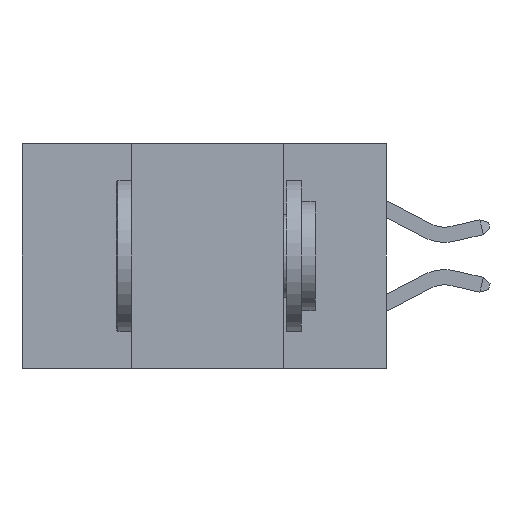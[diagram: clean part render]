
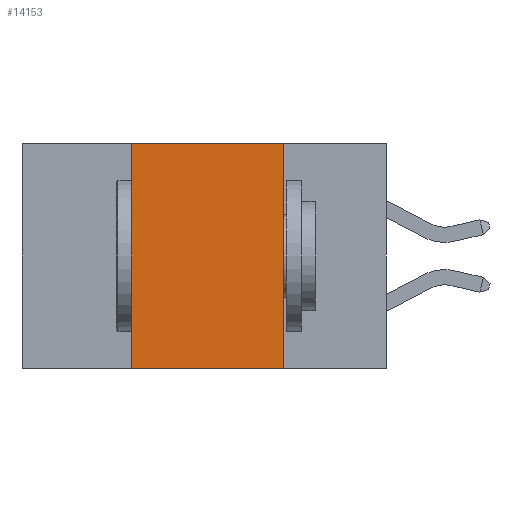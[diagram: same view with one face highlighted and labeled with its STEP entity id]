
A CAD part, left-side view. The second image highlights one B-rep face of the part: STEP entity #14153.
In plain terms, the highlighted planar face has unit normal (-1, 0, 0).
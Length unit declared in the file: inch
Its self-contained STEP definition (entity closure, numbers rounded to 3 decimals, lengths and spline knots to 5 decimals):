
#188 = EDGE_CURVE ( 'NONE', #4220, #5410, #13571, .T. ) ;
#332 = EDGE_CURVE ( 'NONE', #10533, #4220, #10446, .T. ) ;
#414 = EDGE_CURVE ( 'NONE', #7069, #10533, #2718, .T. ) ;
#447 = FACE_OUTER_BOUND ( 'NONE', #1345, .T. ) ;
#1023 = VECTOR ( 'NONE', #4524, 39.37008 ) ;
#1334 = CARTESIAN_POINT ( 'NONE',  ( 0., 0.6, -0.37 ) ) ;
#1345 = EDGE_LOOP ( 'NONE', ( #13591, #1482, #13916, #5212 ) ) ;
#1397 = VECTOR ( 'NONE', #14164, 39.37008 ) ;
#1482 = ORIENTED_EDGE ( 'NONE', *, *, #332, .F. ) ;
#1940 = CARTESIAN_POINT ( 'NONE',  ( 0., 0.42, -0.37 ) ) ;
#2455 = DIRECTION ( 'NONE',  ( 0., 0., -1. ) ) ;
#2718 = LINE ( 'NONE', #1940, #11672 ) ;
#3185 = DIRECTION ( 'NONE',  ( 0., 0., 1. ) ) ;
#4220 = VERTEX_POINT ( 'NONE', #9955 ) ;
#4524 = DIRECTION ( 'NONE',  ( 0., 0., -1. ) ) ;
#5212 = ORIENTED_EDGE ( 'NONE', *, *, #7591, .T. ) ;
#5410 = VERTEX_POINT ( 'NONE', #6975 ) ;
#5785 = CARTESIAN_POINT ( 'NONE',  ( 0., 0.42, -0.37 ) ) ;
#6232 = DIRECTION ( 'NONE',  ( 0., -1., 0. ) ) ;
#6975 = CARTESIAN_POINT ( 'NONE',  ( 0., 0.17, -0.37 ) ) ;
#7069 = VERTEX_POINT ( 'NONE', #5785 ) ;
#7591 = EDGE_CURVE ( 'NONE', #7069, #5410, #10942, .T. ) ;
#8428 = CARTESIAN_POINT ( 'NONE',  ( 0., 0.6, 0. ) ) ;
#9489 = AXIS2_PLACEMENT_3D ( 'NONE', #13929, #9603, #2455 ) ;
#9603 = DIRECTION ( 'NONE',  ( 1., 0., 0. ) ) ;
#9955 = CARTESIAN_POINT ( 'NONE',  ( 0., 0.17, 0. ) ) ;
#10446 = LINE ( 'NONE', #8428, #13728 ) ;
#10533 = VERTEX_POINT ( 'NONE', #13355 ) ;
#10942 = LINE ( 'NONE', #1334, #1397 ) ;
#11026 = CARTESIAN_POINT ( 'NONE',  ( 0., 0.17, -0.37 ) ) ;
#11672 = VECTOR ( 'NONE', #3185, 39.37008 ) ;
#13355 = CARTESIAN_POINT ( 'NONE',  ( 0., 0.42, 0. ) ) ;
#13571 = LINE ( 'NONE', #11026, #1023 ) ;
#13591 = ORIENTED_EDGE ( 'NONE', *, *, #188, .F. ) ;
#13728 = VECTOR ( 'NONE', #6232, 39.37008 ) ;
#13916 = ORIENTED_EDGE ( 'NONE', *, *, #414, .F. ) ;
#13929 = CARTESIAN_POINT ( 'NONE',  ( 0., 0.6, 0. ) ) ;
#13982 = PLANE ( 'NONE',  #9489 ) ;
#14153 = ADVANCED_FACE ( 'NONE', ( #447 ), #13982, .F. ) ;
#14164 = DIRECTION ( 'NONE',  ( 0., -1., 0. ) ) ;
